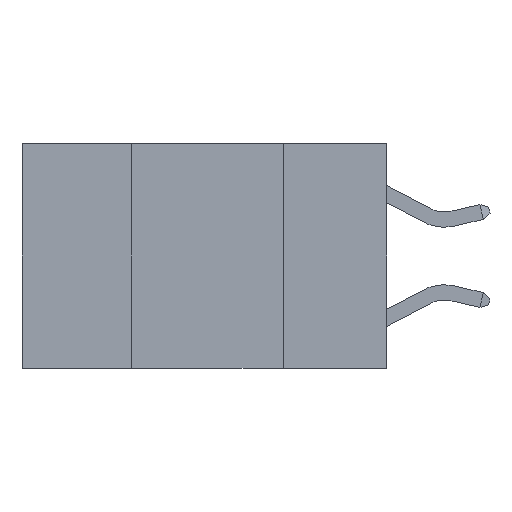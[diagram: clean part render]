
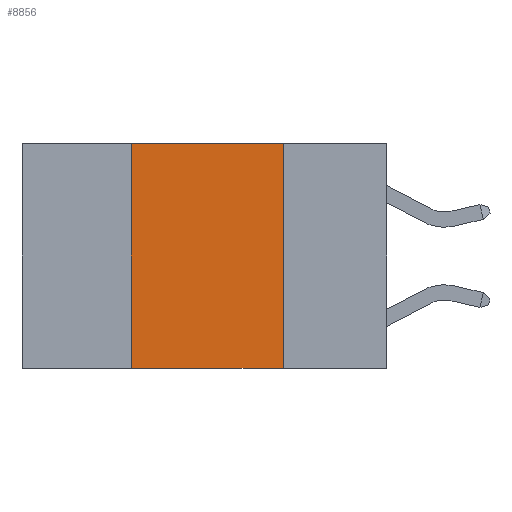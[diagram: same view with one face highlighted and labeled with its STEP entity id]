
A CAD part, left-side view. The second image highlights one B-rep face of the part: STEP entity #8856.
In plain terms, the highlighted planar face has unit normal (-1, 0, 0).
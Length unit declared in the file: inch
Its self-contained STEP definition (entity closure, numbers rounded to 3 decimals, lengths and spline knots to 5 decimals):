
#661 = VECTOR ( 'NONE', #6827, 39.37008 ) ;
#2018 = CARTESIAN_POINT ( 'NONE',  ( 0., 0.42, 0. ) ) ;
#2255 = EDGE_CURVE ( 'NONE', #6823, #6159, #6357, .T. ) ;
#2262 = DIRECTION ( 'NONE',  ( 1., 0., 0. ) ) ;
#2550 = CARTESIAN_POINT ( 'NONE',  ( 0., 0.6, -0.37 ) ) ;
#2679 = EDGE_CURVE ( 'NONE', #6823, #3689, #7233, .T. ) ;
#2829 = CARTESIAN_POINT ( 'NONE',  ( 0., 0.42, 0. ) ) ;
#3054 = ORIENTED_EDGE ( 'NONE', *, *, #2679, .T. ) ;
#3457 = VECTOR ( 'NONE', #3733, 39.37008 ) ;
#3689 = VERTEX_POINT ( 'NONE', #8995 ) ;
#3733 = DIRECTION ( 'NONE',  ( 0., -1., 0. ) ) ;
#3860 = VECTOR ( 'NONE', #10514, 39.37008 ) ;
#3950 = CARTESIAN_POINT ( 'NONE',  ( 0., 0.42, -0.37 ) ) ;
#3993 = FACE_OUTER_BOUND ( 'NONE', #4869, .T. ) ;
#4869 = EDGE_LOOP ( 'NONE', ( #8875, #8056, #8087, #3054 ) ) ;
#4948 = EDGE_CURVE ( 'NONE', #6159, #7494, #5729, .T. ) ;
#5144 = EDGE_CURVE ( 'NONE', #7494, #3689, #6135, .T. ) ;
#5729 = LINE ( 'NONE', #8743, #3457 ) ;
#6135 = LINE ( 'NONE', #9700, #3860 ) ;
#6159 = VERTEX_POINT ( 'NONE', #2018 ) ;
#6280 = DIRECTION ( 'NONE',  ( 0., 0., 1. ) ) ;
#6357 = LINE ( 'NONE', #2829, #8276 ) ;
#6823 = VERTEX_POINT ( 'NONE', #3950 ) ;
#6827 = DIRECTION ( 'NONE',  ( 0., -1., 0. ) ) ;
#7233 = LINE ( 'NONE', #2550, #661 ) ;
#7331 = CARTESIAN_POINT ( 'NONE',  ( 0., 0.17, 0. ) ) ;
#7371 = CARTESIAN_POINT ( 'NONE',  ( 0., 0.6, 0. ) ) ;
#7494 = VERTEX_POINT ( 'NONE', #7331 ) ;
#8056 = ORIENTED_EDGE ( 'NONE', *, *, #4948, .F. ) ;
#8087 = ORIENTED_EDGE ( 'NONE', *, *, #2255, .F. ) ;
#8180 = DIRECTION ( 'NONE',  ( 0., 0., -1. ) ) ;
#8276 = VECTOR ( 'NONE', #6280, 39.37008 ) ;
#8743 = CARTESIAN_POINT ( 'NONE',  ( 0., 0.6, 0. ) ) ;
#8856 = ADVANCED_FACE ( 'NONE', ( #3993 ), #9746, .F. ) ;
#8875 = ORIENTED_EDGE ( 'NONE', *, *, #5144, .F. ) ;
#8918 = AXIS2_PLACEMENT_3D ( 'NONE', #7371, #2262, #8180 ) ;
#8995 = CARTESIAN_POINT ( 'NONE',  ( 0., 0.17, -0.37 ) ) ;
#9700 = CARTESIAN_POINT ( 'NONE',  ( 0., 0.17, 0. ) ) ;
#9746 = PLANE ( 'NONE',  #8918 ) ;
#10514 = DIRECTION ( 'NONE',  ( 0., 0., -1. ) ) ;
